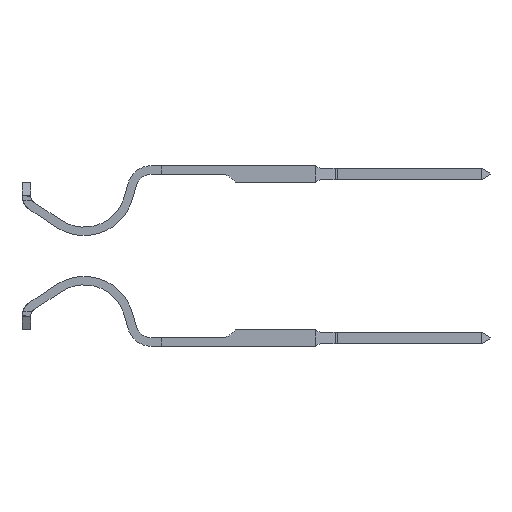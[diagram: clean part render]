
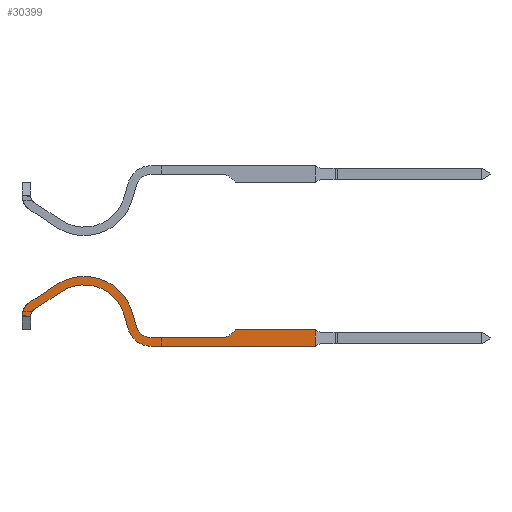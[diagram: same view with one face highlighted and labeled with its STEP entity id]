
A CAD part, left-side view. The second image highlights one B-rep face of the part: STEP entity #30399.
In plain terms, the highlighted face is planar.
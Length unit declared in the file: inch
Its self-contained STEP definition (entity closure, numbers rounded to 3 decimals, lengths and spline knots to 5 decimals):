
#452 = CARTESIAN_POINT ( 'NONE',  ( 0.33, 0.0255, 0.025 ) ) ;
#983 = CARTESIAN_POINT ( 'NONE',  ( 0.15231, 0.06879, 0.025 ) ) ;
#1328 = PLANE ( 'NONE',  #2189 ) ;
#1440 = VECTOR ( 'NONE', #2230, 39.37008 ) ;
#1659 = ORIENTED_EDGE ( 'NONE', *, *, #14025, .T. ) ;
#1795 = CARTESIAN_POINT ( 'NONE',  ( 0.45821, 0.0375, 0.025 ) ) ;
#1886 = CARTESIAN_POINT ( 'NONE',  ( 0.14622, 0.058, 0.025 ) ) ;
#1964 = ORIENTED_EDGE ( 'NONE', *, *, #20937, .F. ) ;
#2116 = EDGE_CURVE ( 'NONE', #12807, #16645, #2381, .T. ) ;
#2189 = AXIS2_PLACEMENT_3D ( 'NONE', #16239, #18768, #3895 ) ;
#2230 = DIRECTION ( 'NONE',  ( 0.268, -0.963, 0. ) ) ;
#2337 = VECTOR ( 'NONE', #30497, 39.37008 ) ;
#2381 = CIRCLE ( 'NONE', #6958, 0.0265 ) ;
#2396 = DIRECTION ( 'NONE',  ( 1., 0., 0. ) ) ;
#2439 = VERTEX_POINT ( 'NONE', #1886 ) ;
#2489 = AXIS2_PLACEMENT_3D ( 'NONE', #24385, #9609, #26846 ) ;
#2644 = VECTOR ( 'NONE', #20678, 39.37008 ) ;
#2870 = LINE ( 'NONE', #14663, #7978 ) ;
#3141 = CARTESIAN_POINT ( 'NONE',  ( 0.43721, 0.04723, 0.025 ) ) ;
#3312 = VERTEX_POINT ( 'NONE', #4942 ) ;
#3500 = AXIS2_PLACEMENT_3D ( 'NONE', #29498, #14753, #31775 ) ;
#3516 = ORIENTED_EDGE ( 'NONE', *, *, #10792, .T. ) ;
#3895 = DIRECTION ( 'NONE',  ( -1., 0., 0. ) ) ;
#3978 = EDGE_CURVE ( 'NONE', #12552, #3312, #7430, .T. ) ;
#4356 = DIRECTION ( 'NONE',  ( -1., 0., 0. ) ) ;
#4543 = CIRCLE ( 'NONE', #3500, 0.0765 ) ;
#4942 = CARTESIAN_POINT ( 'NONE',  ( 0.33, 0.0255, 0.025 ) ) ;
#4943 = CARTESIAN_POINT ( 'NONE',  ( 0.29484, 0.0392, 0.025 ) ) ;
#5029 = CARTESIAN_POINT ( 'NONE',  ( 0.58021, 0.0125, 0.025 ) ) ;
#5091 = VERTEX_POINT ( 'NONE', #18728 ) ;
#5402 = VERTEX_POINT ( 'NONE', #15298 ) ;
#5415 = CARTESIAN_POINT ( 'NONE',  ( 0.43721, 0.0255, 0.025 ) ) ;
#5676 = DIRECTION ( 'NONE',  ( 1., 0., 0. ) ) ;
#6645 = VERTEX_POINT ( 'NONE', #28603 ) ;
#6958 = AXIS2_PLACEMENT_3D ( 'NONE', #20701, #9614, #12392 ) ;
#7430 = CIRCLE ( 'NONE', #23766, 0.0235 ) ;
#7479 = VERTEX_POINT ( 'NONE', #4943 ) ;
#7652 = DIRECTION ( 'NONE',  ( 0.836, 0.549, 0. ) ) ;
#7978 = VECTOR ( 'NONE', #17196, 39.37008 ) ;
#8512 = CARTESIAN_POINT ( 'NONE',  ( 0.13322, 0.058, 0.025 ) ) ;
#8623 = CARTESIAN_POINT ( 'NONE',  ( 0.18604, 0.10646, 0.025 ) ) ;
#8637 = VECTOR ( 'NONE', #24755, 39.37008 ) ;
#8963 = FACE_OUTER_BOUND ( 'NONE', #22506, .T. ) ;
#9609 = DIRECTION ( 'NONE',  ( 0., 0., -1. ) ) ;
#9614 = DIRECTION ( 'NONE',  ( 0., 0., -1. ) ) ;
#9687 = ORIENTED_EDGE ( 'NONE', *, *, #16203, .T. ) ;
#9821 = EDGE_CURVE ( 'NONE', #5402, #14399, #11464, .T. ) ;
#10036 = DIRECTION ( 'NONE',  ( 0., 0., 1. ) ) ;
#10112 = VERTEX_POINT ( 'NONE', #11985 ) ;
#10125 = AXIS2_PLACEMENT_3D ( 'NONE', #31780, #17305, #2396 ) ;
#10792 = EDGE_CURVE ( 'NONE', #2439, #5402, #30210, .T. ) ;
#10799 = LINE ( 'NONE', #22465, #23932 ) ;
#10971 = VERTEX_POINT ( 'NONE', #12592 ) ;
#11105 = VERTEX_POINT ( 'NONE', #8623 ) ;
#11237 = ORIENTED_EDGE ( 'NONE', *, *, #27065, .T. ) ;
#11464 = LINE ( 'NONE', #983, #18071 ) ;
#11825 = VERTEX_POINT ( 'NONE', #17568 ) ;
#11985 = CARTESIAN_POINT ( 'NONE',  ( 0.58021, 0.0375, 0.025 ) ) ;
#12069 = CIRCLE ( 'NONE', #23905, 0.0635 ) ;
#12094 = EDGE_CURVE ( 'NONE', #14399, #11825, #12069, .T. ) ;
#12392 = DIRECTION ( 'NONE',  ( -1., 0., 0. ) ) ;
#12439 = CARTESIAN_POINT ( 'NONE',  ( 0.33, 0.0125, 0.025 ) ) ;
#12552 = VERTEX_POINT ( 'NONE', #29711 ) ;
#12592 = CARTESIAN_POINT ( 'NONE',  ( 0.30169, 0.06304, 0.025 ) ) ;
#12807 = VERTEX_POINT ( 'NONE', #8512 ) ;
#13270 = ORIENTED_EDGE ( 'NONE', *, *, #14898, .F. ) ;
#13491 = CARTESIAN_POINT ( 'NONE',  ( 0.228, 0.0425, 0.025 ) ) ;
#14025 = EDGE_CURVE ( 'NONE', #12807, #2439, #22466, .T. ) ;
#14399 = VERTEX_POINT ( 'NONE', #14553 ) ;
#14553 = CARTESIAN_POINT ( 'NONE',  ( 0.19317, 0.09559, 0.025 ) ) ;
#14663 = CARTESIAN_POINT ( 'NONE',  ( 0.58021, 0.016, 0.025 ) ) ;
#14749 = LINE ( 'NONE', #28134, #2337 ) ;
#14753 = DIRECTION ( 'NONE',  ( 0., 0., -1. ) ) ;
#14898 = EDGE_CURVE ( 'NONE', #16645, #11105, #10799, .T. ) ;
#15200 = CARTESIAN_POINT ( 'NONE',  ( 0.45821, 0.0375, 0.025 ) ) ;
#15298 = CARTESIAN_POINT ( 'NONE',  ( 0.15231, 0.06879, 0.025 ) ) ;
#15844 = ORIENTED_EDGE ( 'NONE', *, *, #9821, .T. ) ;
#15984 = DIRECTION ( 'NONE',  ( -1., 0., 0. ) ) ;
#16203 = EDGE_CURVE ( 'NONE', #25140, #10112, #2870, .T. ) ;
#16239 = CARTESIAN_POINT ( 'NONE',  ( 0.095, 0.025, 0.025 ) ) ;
#16403 = LINE ( 'NONE', #1795, #28715 ) ;
#16517 = ORIENTED_EDGE ( 'NONE', *, *, #3978, .F. ) ;
#16645 = VERTEX_POINT ( 'NONE', #31489 ) ;
#16976 = EDGE_CURVE ( 'NONE', #6645, #21782, #19168, .T. ) ;
#17096 = ORIENTED_EDGE ( 'NONE', *, *, #17338, .T. ) ;
#17196 = DIRECTION ( 'NONE',  ( 0., 1., 0. ) ) ;
#17305 = DIRECTION ( 'NONE',  ( 0., 0., 1. ) ) ;
#17338 = EDGE_CURVE ( 'NONE', #10112, #5091, #16403, .T. ) ;
#17568 = CARTESIAN_POINT ( 'NONE',  ( 0.28917, 0.05955, 0.025 ) ) ;
#18071 = VECTOR ( 'NONE', #28180, 39.37008 ) ;
#18211 = CARTESIAN_POINT ( 'NONE',  ( 0.14621, 0.058, 0.025 ) ) ;
#18229 = ORIENTED_EDGE ( 'NONE', *, *, #2116, .F. ) ;
#18374 = VECTOR ( 'NONE', #20469, 39.37008 ) ;
#18728 = CARTESIAN_POINT ( 'NONE',  ( 0.45821, 0.0375, 0.025 ) ) ;
#18768 = DIRECTION ( 'NONE',  ( 0., 0., -1. ) ) ;
#19168 = CIRCLE ( 'NONE', #25230, 0.02173 ) ;
#19636 = EDGE_CURVE ( 'NONE', #10971, #12552, #22069, .T. ) ;
#19927 = ORIENTED_EDGE ( 'NONE', *, *, #24446, .T. ) ;
#20043 = ORIENTED_EDGE ( 'NONE', *, *, #23847, .F. ) ;
#20134 = VERTEX_POINT ( 'NONE', #26377 ) ;
#20469 = DIRECTION ( 'NONE',  ( 1., 0., 0. ) ) ;
#20510 = DIRECTION ( 'NONE',  ( 0., 0., -1. ) ) ;
#20678 = DIRECTION ( 'NONE',  ( 1., 0., 0. ) ) ;
#20701 = CARTESIAN_POINT ( 'NONE',  ( 0.15971, 0.0575, 0.025 ) ) ;
#20937 = EDGE_CURVE ( 'NONE', #11105, #10971, #4543, .T. ) ;
#21782 = VERTEX_POINT ( 'NONE', #5415 ) ;
#22069 = LINE ( 'NONE', #29350, #1440 ) ;
#22344 = EDGE_CURVE ( 'NONE', #5091, #6645, #23075, .T. ) ;
#22465 = CARTESIAN_POINT ( 'NONE',  ( 0.14518, 0.07966, 0.025 ) ) ;
#22466 = LINE ( 'NONE', #18211, #2644 ) ;
#22506 = EDGE_LOOP ( 'NONE', ( #18229, #1659, #3516, #15844, #24973, #27003, #11237, #19927, #9687, #17096, #25162, #31126, #20043, #16517, #24046, #1964, #13270 ) ) ;
#22560 = LINE ( 'NONE', #12439, #8637 ) ;
#23075 = LINE ( 'NONE', #15200, #29545 ) ;
#23766 = AXIS2_PLACEMENT_3D ( 'NONE', #24800, #10036, #27251 ) ;
#23847 = EDGE_CURVE ( 'NONE', #3312, #21782, #24894, .T. ) ;
#23905 = AXIS2_PLACEMENT_3D ( 'NONE', #13491, #30641, #15984 ) ;
#23932 = VECTOR ( 'NONE', #7652, 39.37008 ) ;
#24046 = ORIENTED_EDGE ( 'NONE', *, *, #19636, .F. ) ;
#24385 = CARTESIAN_POINT ( 'NONE',  ( 0.15971, 0.0575, 0.025 ) ) ;
#24446 = EDGE_CURVE ( 'NONE', #20134, #25140, #22560, .T. ) ;
#24630 = DIRECTION ( 'NONE',  ( -0.707, -0.707, 0. ) ) ;
#24755 = DIRECTION ( 'NONE',  ( 1., 0., 0. ) ) ;
#24800 = CARTESIAN_POINT ( 'NONE',  ( 0.33, 0.049, 0.025 ) ) ;
#24894 = LINE ( 'NONE', #452, #18374 ) ;
#24973 = ORIENTED_EDGE ( 'NONE', *, *, #12094, .T. ) ;
#25140 = VERTEX_POINT ( 'NONE', #5029 ) ;
#25162 = ORIENTED_EDGE ( 'NONE', *, *, #22344, .T. ) ;
#25230 = AXIS2_PLACEMENT_3D ( 'NONE', #3141, #20510, #5676 ) ;
#25389 = EDGE_CURVE ( 'NONE', #11825, #7479, #14749, .T. ) ;
#25864 = CIRCLE ( 'NONE', #10125, 0.0365 ) ;
#26377 = CARTESIAN_POINT ( 'NONE',  ( 0.33, 0.0125, 0.025 ) ) ;
#26846 = DIRECTION ( 'NONE',  ( -1., 0., 0. ) ) ;
#27003 = ORIENTED_EDGE ( 'NONE', *, *, #25389, .T. ) ;
#27065 = EDGE_CURVE ( 'NONE', #7479, #20134, #25864, .T. ) ;
#27251 = DIRECTION ( 'NONE',  ( 1., 0., 0. ) ) ;
#28134 = CARTESIAN_POINT ( 'NONE',  ( 0.28917, 0.05955, 0.025 ) ) ;
#28180 = DIRECTION ( 'NONE',  ( 0.836, 0.549, 0. ) ) ;
#28603 = CARTESIAN_POINT ( 'NONE',  ( 0.45258, 0.03186, 0.025 ) ) ;
#28715 = VECTOR ( 'NONE', #4356, 39.37008 ) ;
#29350 = CARTESIAN_POINT ( 'NONE',  ( 0.30169, 0.06304, 0.025 ) ) ;
#29498 = CARTESIAN_POINT ( 'NONE',  ( 0.228, 0.0425, 0.025 ) ) ;
#29545 = VECTOR ( 'NONE', #24630, 39.37008 ) ;
#29711 = CARTESIAN_POINT ( 'NONE',  ( 0.30736, 0.04269, 0.025 ) ) ;
#30210 = CIRCLE ( 'NONE', #2489, 0.0135 ) ;
#30399 = ADVANCED_FACE ( 'NONE', ( #8963 ), #1328, .F. ) ;
#30497 = DIRECTION ( 'NONE',  ( 0.268, -0.963, 0. ) ) ;
#30641 = DIRECTION ( 'NONE',  ( 0., 0., -1. ) ) ;
#31126 = ORIENTED_EDGE ( 'NONE', *, *, #16976, .T. ) ;
#31489 = CARTESIAN_POINT ( 'NONE',  ( 0.14518, 0.07966, 0.025 ) ) ;
#31775 = DIRECTION ( 'NONE',  ( -1., 0., 0. ) ) ;
#31780 = CARTESIAN_POINT ( 'NONE',  ( 0.33, 0.049, 0.025 ) ) ;
